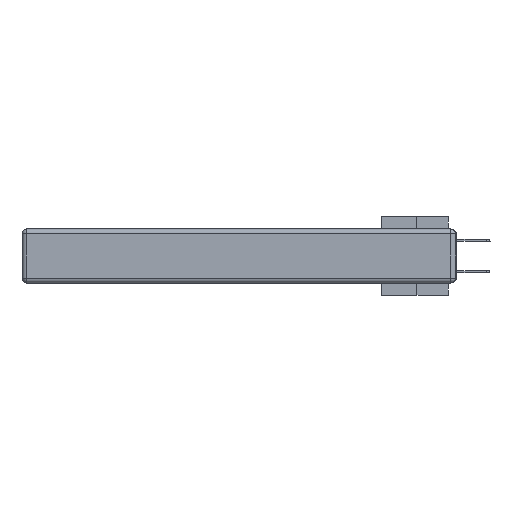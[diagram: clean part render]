
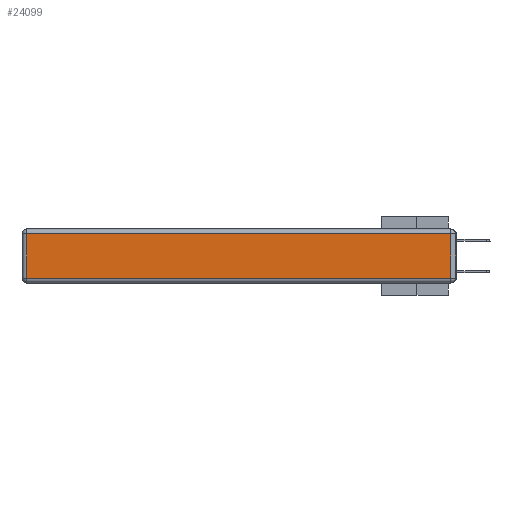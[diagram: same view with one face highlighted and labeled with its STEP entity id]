
A CAD part, left-side view. The second image highlights one B-rep face of the part: STEP entity #24099.
In plain terms, the highlighted planar face has unit normal (-1, 0, 0).
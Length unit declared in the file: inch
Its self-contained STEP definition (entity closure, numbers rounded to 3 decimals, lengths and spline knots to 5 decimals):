
#374 = VECTOR ( 'NONE', #11918, 39.37008 ) ;
#1042 = VECTOR ( 'NONE', #20603, 39.37008 ) ;
#1427 = LINE ( 'NONE', #22650, #1042 ) ;
#3875 = CARTESIAN_POINT ( 'NONE',  ( 0., 2.72, -0.03 ) ) ;
#4516 = DIRECTION ( 'NONE',  ( 0., 0., 1. ) ) ;
#5287 = EDGE_CURVE ( 'NONE', #10220, #24871, #12154, .T. ) ;
#5439 = CARTESIAN_POINT ( 'NONE',  ( 0., 0., -0.313 ) ) ;
#7033 = EDGE_CURVE ( 'NONE', #19091, #10220, #19352, .T. ) ;
#7315 = DIRECTION ( 'NONE',  ( 0., 0., -1. ) ) ;
#8282 = CARTESIAN_POINT ( 'NONE',  ( 0., 0.03, -0.03 ) ) ;
#9012 = PLANE ( 'NONE',  #9419 ) ;
#9419 = AXIS2_PLACEMENT_3D ( 'NONE', #25266, #30020, #4516 ) ;
#9885 = CARTESIAN_POINT ( 'NONE',  ( 0., 2.75, -0.03 ) ) ;
#10220 = VERTEX_POINT ( 'NONE', #3875 ) ;
#11918 = DIRECTION ( 'NONE',  ( 0., 1., 0. ) ) ;
#12154 = LINE ( 'NONE', #21664, #12899 ) ;
#12468 = DIRECTION ( 'NONE',  ( 0., -1., 0. ) ) ;
#12899 = VECTOR ( 'NONE', #7315, 39.37008 ) ;
#13435 = LINE ( 'NONE', #5439, #25785 ) ;
#13512 = EDGE_CURVE ( 'NONE', #24871, #17356, #13435, .T. ) ;
#14497 = ORIENTED_EDGE ( 'NONE', *, *, #5287, .T. ) ;
#14629 = CARTESIAN_POINT ( 'NONE',  ( 0., 2.72, -0.313 ) ) ;
#17106 = EDGE_LOOP ( 'NONE', ( #20973, #18836, #23345, #14497 ) ) ;
#17356 = VERTEX_POINT ( 'NONE', #27929 ) ;
#17871 = EDGE_CURVE ( 'NONE', #17356, #19091, #1427, .T. ) ;
#18836 = ORIENTED_EDGE ( 'NONE', *, *, #17871, .T. ) ;
#19091 = VERTEX_POINT ( 'NONE', #8282 ) ;
#19352 = LINE ( 'NONE', #9885, #374 ) ;
#20603 = DIRECTION ( 'NONE',  ( 0., 0., 1. ) ) ;
#20973 = ORIENTED_EDGE ( 'NONE', *, *, #13512, .T. ) ;
#21664 = CARTESIAN_POINT ( 'NONE',  ( 0., 2.72, -0.343 ) ) ;
#22650 = CARTESIAN_POINT ( 'NONE',  ( 0., 0.03, -0.343 ) ) ;
#23345 = ORIENTED_EDGE ( 'NONE', *, *, #7033, .T. ) ;
#23769 = FACE_OUTER_BOUND ( 'NONE', #17106, .T. ) ;
#24099 = ADVANCED_FACE ( 'NONE', ( #23769 ), #9012, .T. ) ;
#24871 = VERTEX_POINT ( 'NONE', #14629 ) ;
#25266 = CARTESIAN_POINT ( 'NONE',  ( 0., 0., -0.343 ) ) ;
#25785 = VECTOR ( 'NONE', #12468, 39.37008 ) ;
#27929 = CARTESIAN_POINT ( 'NONE',  ( 0., 0.03, -0.313 ) ) ;
#30020 = DIRECTION ( 'NONE',  ( -1., 0., 0. ) ) ;
